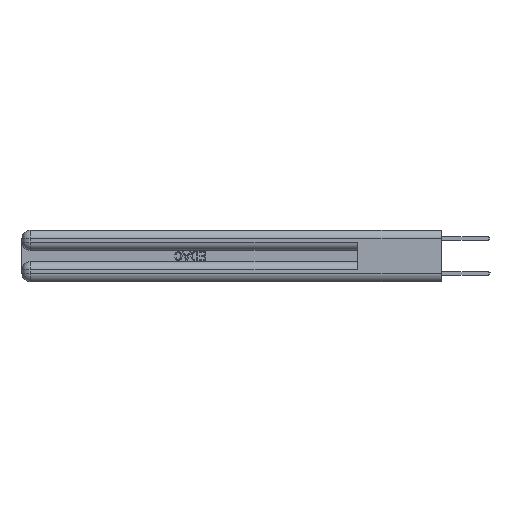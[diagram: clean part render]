
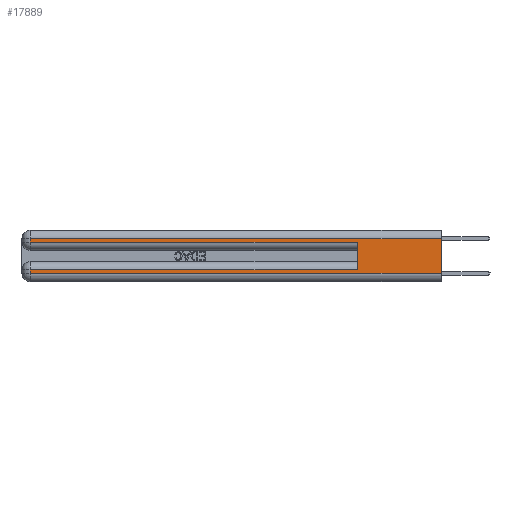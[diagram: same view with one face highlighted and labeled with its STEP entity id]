
A CAD part, left-side view. The second image highlights one B-rep face of the part: STEP entity #17889.
In plain terms, the highlighted planar face has unit normal (-1, 0, 0).
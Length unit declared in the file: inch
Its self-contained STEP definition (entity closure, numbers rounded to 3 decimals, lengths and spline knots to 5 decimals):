
#329 = VECTOR ( 'NONE', #10001, 39.37008 ) ;
#388 = ORIENTED_EDGE ( 'NONE', *, *, #20742, .T. ) ;
#1518 = CARTESIAN_POINT ( 'NONE',  ( 0., 2.94, 0.37 ) ) ;
#2130 = EDGE_CURVE ( 'NONE', #4689, #11375, #15173, .T. ) ;
#4124 = EDGE_LOOP ( 'NONE', ( #7454, #20032, #28349, #16112, #31137, #12264, #388, #10950 ) ) ;
#4405 = CARTESIAN_POINT ( 'NONE',  ( 0., 0.6, 0.285 ) ) ;
#4689 = VERTEX_POINT ( 'NONE', #12873 ) ;
#5290 = VERTEX_POINT ( 'NONE', #9715 ) ;
#5506 = CARTESIAN_POINT ( 'NONE',  ( 0., 0.6, 0.145 ) ) ;
#6416 = VECTOR ( 'NONE', #18328, 39.37008 ) ;
#6482 = VECTOR ( 'NONE', #30191, 39.37008 ) ;
#6541 = DIRECTION ( 'NONE',  ( 0., 1., 0. ) ) ;
#6627 = DIRECTION ( 'NONE',  ( 0., 1., 0. ) ) ;
#7115 = CARTESIAN_POINT ( 'NONE',  ( 0., 0., 0.37 ) ) ;
#7454 = ORIENTED_EDGE ( 'NONE', *, *, #2130, .F. ) ;
#7865 = VERTEX_POINT ( 'NONE', #27024 ) ;
#8032 = CARTESIAN_POINT ( 'NONE',  ( 0., 0.6, 0.085 ) ) ;
#8515 = VERTEX_POINT ( 'NONE', #8032 ) ;
#8843 = AXIS2_PLACEMENT_3D ( 'NONE', #25812, #31480, #17411 ) ;
#9336 = LINE ( 'NONE', #5506, #21375 ) ;
#9478 = CARTESIAN_POINT ( 'NONE',  ( 0., 2.94, 0.37 ) ) ;
#9715 = CARTESIAN_POINT ( 'NONE',  ( 0., 2.94, 0.085 ) ) ;
#10001 = DIRECTION ( 'NONE',  ( 0., 0., -1. ) ) ;
#10742 = DIRECTION ( 'NONE',  ( 0., 0., 1. ) ) ;
#10950 = ORIENTED_EDGE ( 'NONE', *, *, #31228, .T. ) ;
#10987 = VECTOR ( 'NONE', #6627, 39.37008 ) ;
#11375 = VERTEX_POINT ( 'NONE', #29652 ) ;
#11423 = PLANE ( 'NONE',  #8843 ) ;
#12264 = ORIENTED_EDGE ( 'NONE', *, *, #22795, .T. ) ;
#12873 = CARTESIAN_POINT ( 'NONE',  ( 0., 0., 0.31 ) ) ;
#14920 = CARTESIAN_POINT ( 'NONE',  ( 0., 2.94, 0.06 ) ) ;
#15173 = LINE ( 'NONE', #7115, #21490 ) ;
#15326 = EDGE_CURVE ( 'NONE', #24038, #7865, #29957, .T. ) ;
#16112 = ORIENTED_EDGE ( 'NONE', *, *, #22911, .T. ) ;
#17411 = DIRECTION ( 'NONE',  ( 0., 0., -1. ) ) ;
#17889 = ADVANCED_FACE ( 'NONE', ( #18350 ), #11423, .F. ) ;
#18328 = DIRECTION ( 'NONE',  ( 0., 0., -1. ) ) ;
#18350 = FACE_OUTER_BOUND ( 'NONE', #4124, .T. ) ;
#18405 = EDGE_CURVE ( 'NONE', #4689, #24038, #23177, .T. ) ;
#18464 = CARTESIAN_POINT ( 'NONE',  ( 0., 0., 0.285 ) ) ;
#19814 = DIRECTION ( 'NONE',  ( 0., -1., 0. ) ) ;
#20032 = ORIENTED_EDGE ( 'NONE', *, *, #18405, .T. ) ;
#20138 = VERTEX_POINT ( 'NONE', #14920 ) ;
#20195 = CARTESIAN_POINT ( 'NONE',  ( 0., 0., 0.06 ) ) ;
#20742 = EDGE_CURVE ( 'NONE', #5290, #20138, #28348, .T. ) ;
#21375 = VECTOR ( 'NONE', #10742, 39.37008 ) ;
#21440 = DIRECTION ( 'NONE',  ( 0., 0., -1. ) ) ;
#21490 = VECTOR ( 'NONE', #21440, 39.37008 ) ;
#22023 = VECTOR ( 'NONE', #19814, 39.37008 ) ;
#22795 = EDGE_CURVE ( 'NONE', #8515, #5290, #26992, .T. ) ;
#22911 = EDGE_CURVE ( 'NONE', #7865, #28814, #28237, .T. ) ;
#23177 = LINE ( 'NONE', #34824, #28889 ) ;
#24038 = VERTEX_POINT ( 'NONE', #27522 ) ;
#25812 = CARTESIAN_POINT ( 'NONE',  ( 0., 0., 0.37 ) ) ;
#26373 = CARTESIAN_POINT ( 'NONE',  ( 0., 0., 0.085 ) ) ;
#26992 = LINE ( 'NONE', #26373, #10987 ) ;
#27024 = CARTESIAN_POINT ( 'NONE',  ( 0., 2.94, 0.285 ) ) ;
#27522 = CARTESIAN_POINT ( 'NONE',  ( 0., 2.94, 0.31 ) ) ;
#28237 = LINE ( 'NONE', #18464, #6482 ) ;
#28348 = LINE ( 'NONE', #1518, #329 ) ;
#28349 = ORIENTED_EDGE ( 'NONE', *, *, #15326, .T. ) ;
#28814 = VERTEX_POINT ( 'NONE', #4405 ) ;
#28889 = VECTOR ( 'NONE', #6541, 39.37008 ) ;
#29652 = CARTESIAN_POINT ( 'NONE',  ( 0., 0., 0.06 ) ) ;
#29957 = LINE ( 'NONE', #9478, #6416 ) ;
#30191 = DIRECTION ( 'NONE',  ( 0., -1., 0. ) ) ;
#31137 = ORIENTED_EDGE ( 'NONE', *, *, #34522, .F. ) ;
#31228 = EDGE_CURVE ( 'NONE', #20138, #11375, #35716, .T. ) ;
#31480 = DIRECTION ( 'NONE',  ( 1., 0., 0. ) ) ;
#34522 = EDGE_CURVE ( 'NONE', #8515, #28814, #9336, .T. ) ;
#34824 = CARTESIAN_POINT ( 'NONE',  ( 0., 0., 0.31 ) ) ;
#35716 = LINE ( 'NONE', #20195, #22023 ) ;
